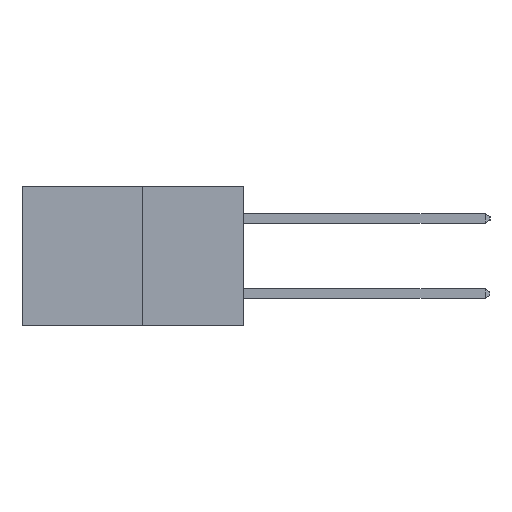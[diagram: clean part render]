
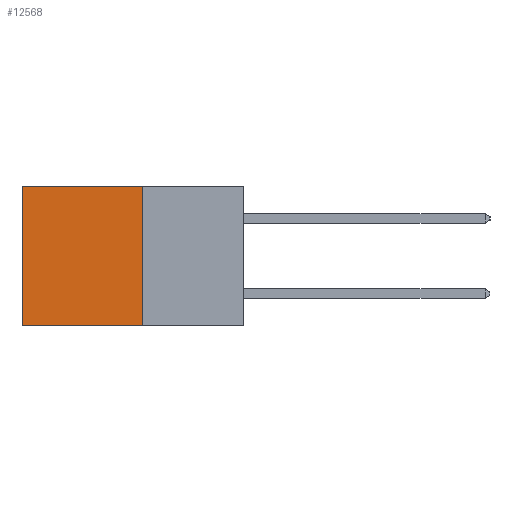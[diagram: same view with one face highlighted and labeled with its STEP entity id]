
A CAD part, left-side view. The second image highlights one B-rep face of the part: STEP entity #12568.
In plain terms, the highlighted planar face has unit normal (-1, 0, 0).
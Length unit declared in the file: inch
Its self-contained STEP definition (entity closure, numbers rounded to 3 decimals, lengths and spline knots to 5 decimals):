
#616 = ORIENTED_EDGE ( 'NONE', *, *, #23703, .F. ) ;
#1093 = CARTESIAN_POINT ( 'NONE',  ( 0.277, 0.59, -0.37 ) ) ;
#1866 = CARTESIAN_POINT ( 'NONE',  ( 0.277, 0.27, 0. ) ) ;
#2062 = FACE_OUTER_BOUND ( 'NONE', #8486, .T. ) ;
#2538 = LINE ( 'NONE', #20471, #3276 ) ;
#3276 = VECTOR ( 'NONE', #25224, 39.37008 ) ;
#6534 = ORIENTED_EDGE ( 'NONE', *, *, #29361, .T. ) ;
#6702 = DIRECTION ( 'NONE',  ( 0., 1., 0. ) ) ;
#8486 = EDGE_LOOP ( 'NONE', ( #6534, #616, #22902, #22857 ) ) ;
#8710 = VECTOR ( 'NONE', #10650, 39.37008 ) ;
#9079 = LINE ( 'NONE', #1866, #20920 ) ;
#10650 = DIRECTION ( 'NONE',  ( 0., 0., -1. ) ) ;
#11918 = CARTESIAN_POINT ( 'NONE',  ( 0.277, 0.27, -0.37 ) ) ;
#12568 = ADVANCED_FACE ( 'NONE', ( #2062 ), #27341, .F. ) ;
#13433 = EDGE_CURVE ( 'NONE', #19727, #22863, #9079, .T. ) ;
#13529 = LINE ( 'NONE', #1093, #8710 ) ;
#15524 = DIRECTION ( 'NONE',  ( 0., 0., -1. ) ) ;
#16266 = VERTEX_POINT ( 'NONE', #17245 ) ;
#17245 = CARTESIAN_POINT ( 'NONE',  ( 0.277, 0.59, -0.37 ) ) ;
#17455 = LINE ( 'NONE', #18514, #22293 ) ;
#17587 = AXIS2_PLACEMENT_3D ( 'NONE', #24941, #29733, #15524 ) ;
#18514 = CARTESIAN_POINT ( 'NONE',  ( 0.277, 0.27, -0.37 ) ) ;
#19727 = VERTEX_POINT ( 'NONE', #29886 ) ;
#20471 = CARTESIAN_POINT ( 'NONE',  ( 0.277, 0.27, -0.37 ) ) ;
#20920 = VECTOR ( 'NONE', #23189, 39.37008 ) ;
#22293 = VECTOR ( 'NONE', #6702, 39.37008 ) ;
#22766 = CARTESIAN_POINT ( 'NONE',  ( 0.277, 0.59, 0. ) ) ;
#22857 = ORIENTED_EDGE ( 'NONE', *, *, #13433, .T. ) ;
#22863 = VERTEX_POINT ( 'NONE', #22766 ) ;
#22902 = ORIENTED_EDGE ( 'NONE', *, *, #25598, .F. ) ;
#23189 = DIRECTION ( 'NONE',  ( 0., 1., 0. ) ) ;
#23703 = EDGE_CURVE ( 'NONE', #25151, #16266, #17455, .T. ) ;
#24941 = CARTESIAN_POINT ( 'NONE',  ( 0.277, 0.27, -0.37 ) ) ;
#25151 = VERTEX_POINT ( 'NONE', #11918 ) ;
#25224 = DIRECTION ( 'NONE',  ( 0., 0., -1. ) ) ;
#25598 = EDGE_CURVE ( 'NONE', #19727, #25151, #2538, .T. ) ;
#27341 = PLANE ( 'NONE',  #17587 ) ;
#29361 = EDGE_CURVE ( 'NONE', #22863, #16266, #13529, .T. ) ;
#29733 = DIRECTION ( 'NONE',  ( 1., 0., 0. ) ) ;
#29886 = CARTESIAN_POINT ( 'NONE',  ( 0.277, 0.27, 0. ) ) ;
